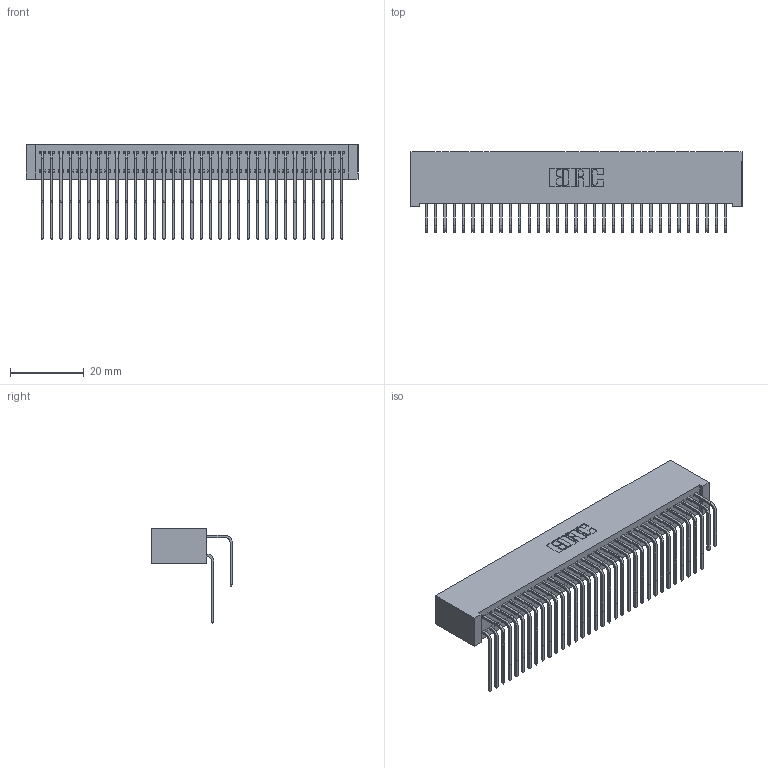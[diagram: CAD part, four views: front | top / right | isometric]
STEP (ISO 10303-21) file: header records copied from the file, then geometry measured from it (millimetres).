
FILE_DESCRIPTION (( 'STEP AP203' ), '1' );
FILE_NAME ('392-066-558-201.STEP', '2018-08-17T22:28:11', ( '' ), ( '' ), 'SwSTEP 2.0', 'SolidWorks 2016', '' );
FILE_SCHEMA (( 'CONFIG_CONTROL_DESIGN' ));
Length unit declared in the file: inch
Products named in the file (4): 345-292-001_558 559 Tail - 1; 345-292-001_558 Tail - 2; 392-066-558-201; 342 Part_Lugless
Assembly tree (67 placements, depth 2):
  392-066-558-201
    342 Part_Lugless
    345-292-001_558 559 Tail - 1  x33
    345-292-001_558 Tail - 2  x33
Bounding box: 90.07 x 21.91 x 25.78 mm (x, y, z)
Volume: 8870.3 mm3; surface area: 16385.4 mm2
Topology: 67 solids, 67 shells, 3666 faces, 10901 edges, 7178 vertices
Faces by surface type: plane 2570, cylinder 1096
Entity records: 23769 total; most frequent: CARTESIAN_POINT 3997, ORIENTED_EDGE 3882, DIRECTION 3405, EDGE_CURVE 1941, VECTOR 1781, LINE 1781, VERTEX_POINT 1290, AXIS2_PLACEMENT_3D 812
